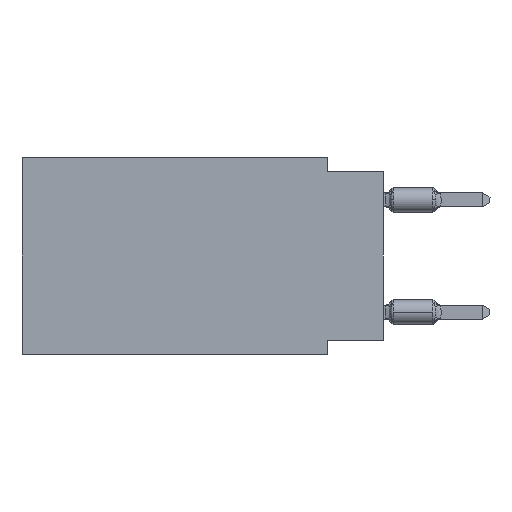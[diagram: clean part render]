
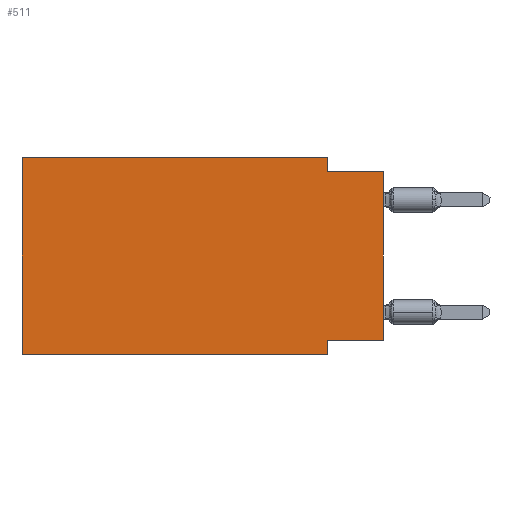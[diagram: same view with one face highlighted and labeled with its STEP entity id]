
A CAD part, left-side view. The second image highlights one B-rep face of the part: STEP entity #511.
In plain terms, the highlighted planar face has unit normal (-1, 0, 0).
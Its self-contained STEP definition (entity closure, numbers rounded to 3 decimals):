
#128 = EDGE_CURVE ( 'NONE', #11949, #11697, #9563, .T. ) ;
#398 = DIRECTION ( 'NONE',  ( 0., 0., -1. ) ) ;
#455 = EDGE_CURVE ( 'NONE', #7325, #8577, #3872, .T. ) ;
#511 = ADVANCED_FACE ( 'NONE', ( #1284 ), #2435, .F. ) ;
#603 = EDGE_CURVE ( 'NONE', #11697, #7325, #5563, .T. ) ;
#815 = VECTOR ( 'NONE', #3382, 1000. ) ;
#1096 = EDGE_CURVE ( 'NONE', #11496, #11949, #6849, .T. ) ;
#1284 = FACE_OUTER_BOUND ( 'NONE', #2439, .T. ) ;
#1382 = DIRECTION ( 'NONE',  ( 0., -1., 0. ) ) ;
#1475 = ORIENTED_EDGE ( 'NONE', *, *, #6253, .T. ) ;
#1635 = AXIS2_PLACEMENT_3D ( 'NONE', #8580, #6594, #10833 ) ;
#1979 = DIRECTION ( 'NONE',  ( 0., 0., -1. ) ) ;
#2232 = LINE ( 'NONE', #2375, #815 ) ;
#2327 = CARTESIAN_POINT ( 'NONE',  ( 0., 16.383, 0. ) ) ;
#2375 = CARTESIAN_POINT ( 'NONE',  ( 0., 16.383, -8.89 ) ) ;
#2433 = ORIENTED_EDGE ( 'NONE', *, *, #11304, .T. ) ;
#2435 = PLANE ( 'NONE',  #1635 ) ;
#2439 = EDGE_LOOP ( 'NONE', ( #2433, #13440, #10067, #4454, #11330, #1475, #13356, #13187 ) ) ;
#2496 = CARTESIAN_POINT ( 'NONE',  ( 0., 2.54, 0. ) ) ;
#2965 = CARTESIAN_POINT ( 'NONE',  ( 0., 2.54, -0.635 ) ) ;
#3116 = DIRECTION ( 'NONE',  ( 0., 0., 1. ) ) ;
#3364 = VECTOR ( 'NONE', #398, 1000. ) ;
#3382 = DIRECTION ( 'NONE',  ( 0., -1., 0. ) ) ;
#3517 = DIRECTION ( 'NONE',  ( 0., 1., 0. ) ) ;
#3757 = DIRECTION ( 'NONE',  ( 0., 0., 1. ) ) ;
#3872 = LINE ( 'NONE', #10239, #8612 ) ;
#4110 = VECTOR ( 'NONE', #3116, 1000. ) ;
#4158 = VERTEX_POINT ( 'NONE', #8687 ) ;
#4362 = CARTESIAN_POINT ( 'NONE',  ( 0., 16.383, 0. ) ) ;
#4454 = ORIENTED_EDGE ( 'NONE', *, *, #128, .F. ) ;
#4781 = CARTESIAN_POINT ( 'NONE',  ( 0., 2.54, 0. ) ) ;
#4999 = VERTEX_POINT ( 'NONE', #13071 ) ;
#5563 = LINE ( 'NONE', #2496, #3364 ) ;
#6253 = EDGE_CURVE ( 'NONE', #11496, #8794, #2232, .T. ) ;
#6594 = DIRECTION ( 'NONE',  ( 1., 0., 0. ) ) ;
#6715 = VECTOR ( 'NONE', #3517, 1000. ) ;
#6723 = CARTESIAN_POINT ( 'NONE',  ( 0., 0., -0.635 ) ) ;
#6849 = LINE ( 'NONE', #8012, #12982 ) ;
#7068 = EDGE_CURVE ( 'NONE', #4999, #4158, #12743, .T. ) ;
#7325 = VERTEX_POINT ( 'NONE', #2965 ) ;
#8012 = CARTESIAN_POINT ( 'NONE',  ( 0., 16.383, 0. ) ) ;
#8197 = LINE ( 'NONE', #11201, #9116 ) ;
#8577 = VERTEX_POINT ( 'NONE', #6723 ) ;
#8580 = CARTESIAN_POINT ( 'NONE',  ( 0., 16.383, 0. ) ) ;
#8612 = VECTOR ( 'NONE', #12484, 1000. ) ;
#8687 = CARTESIAN_POINT ( 'NONE',  ( 0., 2.54, -8.255 ) ) ;
#8794 = VERTEX_POINT ( 'NONE', #9436 ) ;
#9116 = VECTOR ( 'NONE', #1979, 1000. ) ;
#9436 = CARTESIAN_POINT ( 'NONE',  ( 0., 2.54, -8.89 ) ) ;
#9563 = LINE ( 'NONE', #4362, #10989 ) ;
#10067 = ORIENTED_EDGE ( 'NONE', *, *, #603, .F. ) ;
#10120 = EDGE_CURVE ( 'NONE', #4158, #8794, #8197, .T. ) ;
#10239 = CARTESIAN_POINT ( 'NONE',  ( 0., 0., -0.635 ) ) ;
#10365 = CARTESIAN_POINT ( 'NONE',  ( 0., 0., 0. ) ) ;
#10709 = CARTESIAN_POINT ( 'NONE',  ( 0., 0., -8.255 ) ) ;
#10833 = DIRECTION ( 'NONE',  ( 0., 0., -1. ) ) ;
#10989 = VECTOR ( 'NONE', #1382, 1000. ) ;
#11201 = CARTESIAN_POINT ( 'NONE',  ( 0., 2.54, -8.89 ) ) ;
#11304 = EDGE_CURVE ( 'NONE', #4999, #8577, #11388, .T. ) ;
#11330 = ORIENTED_EDGE ( 'NONE', *, *, #1096, .F. ) ;
#11388 = LINE ( 'NONE', #10365, #4110 ) ;
#11496 = VERTEX_POINT ( 'NONE', #13023 ) ;
#11697 = VERTEX_POINT ( 'NONE', #4781 ) ;
#11949 = VERTEX_POINT ( 'NONE', #2327 ) ;
#12484 = DIRECTION ( 'NONE',  ( 0., -1., 0. ) ) ;
#12743 = LINE ( 'NONE', #10709, #6715 ) ;
#12982 = VECTOR ( 'NONE', #3757, 1000. ) ;
#13023 = CARTESIAN_POINT ( 'NONE',  ( 0., 16.383, -8.89 ) ) ;
#13071 = CARTESIAN_POINT ( 'NONE',  ( 0., 0., -8.255 ) ) ;
#13187 = ORIENTED_EDGE ( 'NONE', *, *, #7068, .F. ) ;
#13356 = ORIENTED_EDGE ( 'NONE', *, *, #10120, .F. ) ;
#13440 = ORIENTED_EDGE ( 'NONE', *, *, #455, .F. ) ;
